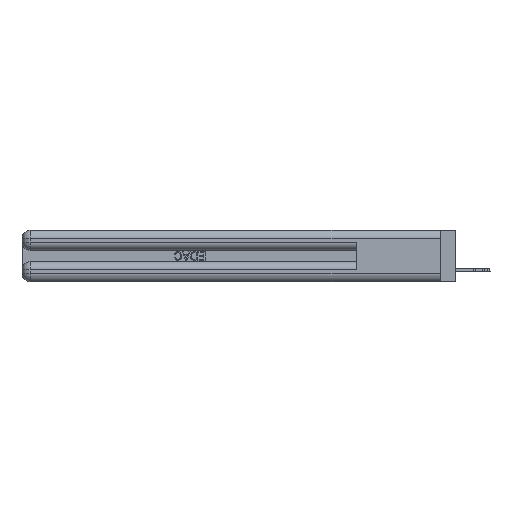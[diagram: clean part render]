
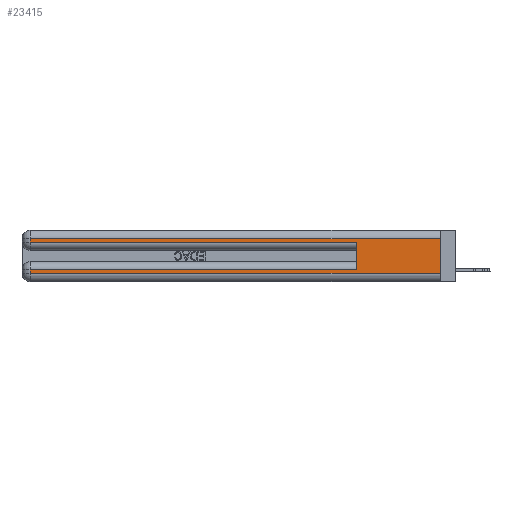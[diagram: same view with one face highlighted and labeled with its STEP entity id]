
A CAD part, left-side view. The second image highlights one B-rep face of the part: STEP entity #23415.
In plain terms, the highlighted planar face has unit normal (-1, 0, 0).
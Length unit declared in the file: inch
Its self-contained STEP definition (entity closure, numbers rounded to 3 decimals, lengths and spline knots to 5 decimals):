
#1120 = CARTESIAN_POINT ( 'NONE',  ( 0., 0.6, 0.145 ) ) ;
#1505 = LINE ( 'NONE', #11489, #43801 ) ;
#1860 = DIRECTION ( 'NONE',  ( 0., 0., 1. ) ) ;
#2960 = CARTESIAN_POINT ( 'NONE',  ( 0., 0.6, 0.085 ) ) ;
#3330 = CARTESIAN_POINT ( 'NONE',  ( 0., 0., 0.31 ) ) ;
#4137 = DIRECTION ( 'NONE',  ( 0., 0., -1. ) ) ;
#4500 = CARTESIAN_POINT ( 'NONE',  ( 0., 0., 0.06 ) ) ;
#4911 = EDGE_CURVE ( 'NONE', #33843, #18604, #1505, .T. ) ;
#6437 = CARTESIAN_POINT ( 'NONE',  ( 0., 0., 0.37 ) ) ;
#8616 = CARTESIAN_POINT ( 'NONE',  ( 0., 0., 0.37 ) ) ;
#8677 = ORIENTED_EDGE ( 'NONE', *, *, #51636, .T. ) ;
#9278 = ORIENTED_EDGE ( 'NONE', *, *, #38267, .F. ) ;
#9304 = VERTEX_POINT ( 'NONE', #2960 ) ;
#11139 = DIRECTION ( 'NONE',  ( 0., -1., 0. ) ) ;
#11489 = CARTESIAN_POINT ( 'NONE',  ( 0., 0., 0.06 ) ) ;
#12236 = DIRECTION ( 'NONE',  ( 0., 0., -1. ) ) ;
#12289 = ORIENTED_EDGE ( 'NONE', *, *, #36761, .F. ) ;
#12746 = CARTESIAN_POINT ( 'NONE',  ( 0., 2.94, 0.285 ) ) ;
#13368 = DIRECTION ( 'NONE',  ( 0., 0., -1. ) ) ;
#15573 = VERTEX_POINT ( 'NONE', #39038 ) ;
#16742 = ORIENTED_EDGE ( 'NONE', *, *, #35638, .T. ) ;
#18604 = VERTEX_POINT ( 'NONE', #4500 ) ;
#21228 = ORIENTED_EDGE ( 'NONE', *, *, #37044, .T. ) ;
#21454 = VECTOR ( 'NONE', #12236, 39.37008 ) ;
#22901 = DIRECTION ( 'NONE',  ( 0., -1., 0. ) ) ;
#23415 = ADVANCED_FACE ( 'NONE', ( #38411 ), #45733, .F. ) ;
#24094 = LINE ( 'NONE', #47434, #52834 ) ;
#24143 = VERTEX_POINT ( 'NONE', #12746 ) ;
#24599 = ORIENTED_EDGE ( 'NONE', *, *, #37614, .T. ) ;
#24684 = VERTEX_POINT ( 'NONE', #46457 ) ;
#25209 = CARTESIAN_POINT ( 'NONE',  ( 0., 2.94, 0.37 ) ) ;
#25676 = EDGE_CURVE ( 'NONE', #36722, #33843, #38840, .T. ) ;
#27403 = VECTOR ( 'NONE', #48016, 39.37008 ) ;
#29279 = LINE ( 'NONE', #1120, #33104 ) ;
#29867 = CARTESIAN_POINT ( 'NONE',  ( 0., 0., 0.31 ) ) ;
#30448 = LINE ( 'NONE', #6437, #21454 ) ;
#30523 = VECTOR ( 'NONE', #13368, 39.37008 ) ;
#33020 = VERTEX_POINT ( 'NONE', #29867 ) ;
#33104 = VECTOR ( 'NONE', #1860, 39.37008 ) ;
#33843 = VERTEX_POINT ( 'NONE', #34188 ) ;
#34188 = CARTESIAN_POINT ( 'NONE',  ( 0., 2.94, 0.06 ) ) ;
#35127 = AXIS2_PLACEMENT_3D ( 'NONE', #8616, #44873, #4137 ) ;
#35587 = CARTESIAN_POINT ( 'NONE',  ( 0., 0., 0.285 ) ) ;
#35638 = EDGE_CURVE ( 'NONE', #15573, #24143, #24094, .T. ) ;
#35739 = DIRECTION ( 'NONE',  ( 0., 1., 0. ) ) ;
#36508 = VECTOR ( 'NONE', #35739, 39.37008 ) ;
#36722 = VERTEX_POINT ( 'NONE', #42412 ) ;
#36761 = EDGE_CURVE ( 'NONE', #9304, #24684, #29279, .T. ) ;
#37044 = EDGE_CURVE ( 'NONE', #33020, #15573, #50979, .T. ) ;
#37614 = EDGE_CURVE ( 'NONE', #24143, #24684, #52914, .T. ) ;
#38267 = EDGE_CURVE ( 'NONE', #33020, #18604, #30448, .T. ) ;
#38411 = FACE_OUTER_BOUND ( 'NONE', #51942, .T. ) ;
#38840 = LINE ( 'NONE', #25209, #30523 ) ;
#39038 = CARTESIAN_POINT ( 'NONE',  ( 0., 2.94, 0.31 ) ) ;
#39177 = DIRECTION ( 'NONE',  ( 0., 0., -1. ) ) ;
#42178 = LINE ( 'NONE', #48093, #36508 ) ;
#42412 = CARTESIAN_POINT ( 'NONE',  ( 0., 2.94, 0.085 ) ) ;
#43801 = VECTOR ( 'NONE', #11139, 39.37008 ) ;
#44611 = VECTOR ( 'NONE', #22901, 39.37008 ) ;
#44873 = DIRECTION ( 'NONE',  ( 1., 0., 0. ) ) ;
#45097 = ORIENTED_EDGE ( 'NONE', *, *, #25676, .T. ) ;
#45733 = PLANE ( 'NONE',  #35127 ) ;
#46457 = CARTESIAN_POINT ( 'NONE',  ( 0., 0.6, 0.285 ) ) ;
#47434 = CARTESIAN_POINT ( 'NONE',  ( 0., 2.94, 0.37 ) ) ;
#48016 = DIRECTION ( 'NONE',  ( 0., 1., 0. ) ) ;
#48093 = CARTESIAN_POINT ( 'NONE',  ( 0., 0., 0.085 ) ) ;
#50979 = LINE ( 'NONE', #3330, #27403 ) ;
#51526 = ORIENTED_EDGE ( 'NONE', *, *, #4911, .T. ) ;
#51636 = EDGE_CURVE ( 'NONE', #9304, #36722, #42178, .T. ) ;
#51942 = EDGE_LOOP ( 'NONE', ( #9278, #21228, #16742, #24599, #12289, #8677, #45097, #51526 ) ) ;
#52834 = VECTOR ( 'NONE', #39177, 39.37008 ) ;
#52914 = LINE ( 'NONE', #35587, #44611 ) ;
